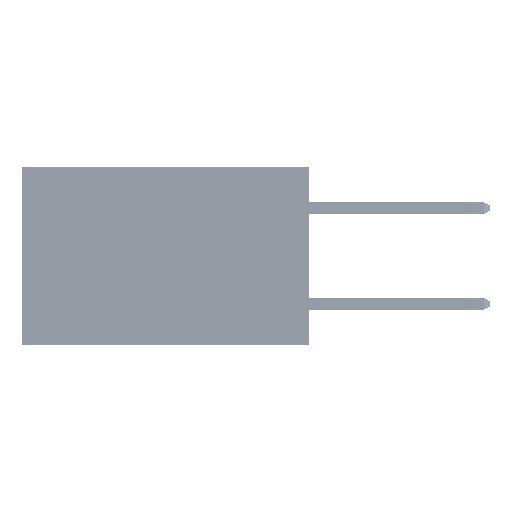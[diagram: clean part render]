
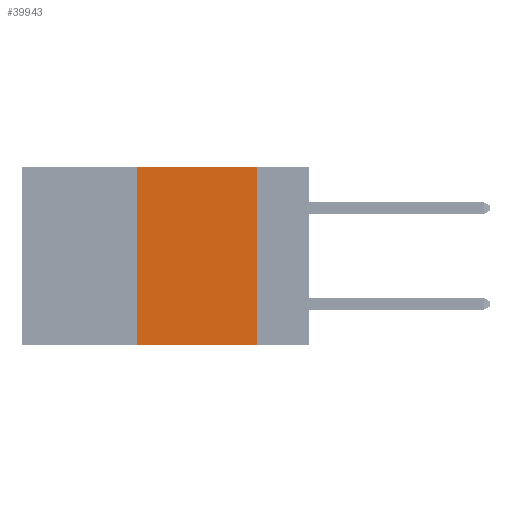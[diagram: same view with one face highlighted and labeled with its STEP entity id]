
A CAD part, left-side view. The second image highlights one B-rep face of the part: STEP entity #39943.
In plain terms, the highlighted planar face has unit normal (-1, 0, 0).
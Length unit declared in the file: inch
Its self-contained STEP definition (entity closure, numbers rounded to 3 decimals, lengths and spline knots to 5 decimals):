
#346 = ORIENTED_EDGE ( 'NONE', *, *, #14190, .F. ) ;
#1102 = VERTEX_POINT ( 'NONE', #16699 ) ;
#1787 = DIRECTION ( 'NONE',  ( 0., 0., -1. ) ) ;
#3929 = AXIS2_PLACEMENT_3D ( 'NONE', #20091, #16231, #43845 ) ;
#5453 = VERTEX_POINT ( 'NONE', #39132 ) ;
#7000 = LINE ( 'NONE', #47631, #37376 ) ;
#9841 = CARTESIAN_POINT ( 'NONE',  ( 0., 0.11, 0. ) ) ;
#10837 = VERTEX_POINT ( 'NONE', #27097 ) ;
#14190 = EDGE_CURVE ( 'NONE', #10837, #29633, #47298, .T. ) ;
#14704 = ORIENTED_EDGE ( 'NONE', *, *, #35596, .T. ) ;
#15706 = DIRECTION ( 'NONE',  ( 0., -1., 0. ) ) ;
#15838 = VECTOR ( 'NONE', #50780, 39.37008 ) ;
#16231 = DIRECTION ( 'NONE',  ( 1., 0., 0. ) ) ;
#16336 = FACE_OUTER_BOUND ( 'NONE', #43054, .T. ) ;
#16699 = CARTESIAN_POINT ( 'NONE',  ( 0., 0.11, -0.37 ) ) ;
#18753 = EDGE_CURVE ( 'NONE', #5453, #10837, #7000, .T. ) ;
#20091 = CARTESIAN_POINT ( 'NONE',  ( 0., 0.6, 0. ) ) ;
#21729 = LINE ( 'NONE', #35399, #30976 ) ;
#24041 = LINE ( 'NONE', #9841, #33251 ) ;
#24071 = ORIENTED_EDGE ( 'NONE', *, *, #18753, .F. ) ;
#25742 = EDGE_CURVE ( 'NONE', #29633, #1102, #24041, .T. ) ;
#27097 = CARTESIAN_POINT ( 'NONE',  ( 0., 0.36, 0. ) ) ;
#29633 = VERTEX_POINT ( 'NONE', #31015 ) ;
#30976 = VECTOR ( 'NONE', #15706, 39.37008 ) ;
#31015 = CARTESIAN_POINT ( 'NONE',  ( 0., 0.11, 0. ) ) ;
#33251 = VECTOR ( 'NONE', #1787, 39.37008 ) ;
#35399 = CARTESIAN_POINT ( 'NONE',  ( 0., 0.6, -0.37 ) ) ;
#35596 = EDGE_CURVE ( 'NONE', #5453, #1102, #21729, .T. ) ;
#35781 = DIRECTION ( 'NONE',  ( 0., 0., 1. ) ) ;
#37376 = VECTOR ( 'NONE', #35781, 39.37008 ) ;
#39132 = CARTESIAN_POINT ( 'NONE',  ( 0., 0.36, -0.37 ) ) ;
#39924 = PLANE ( 'NONE',  #3929 ) ;
#39943 = ADVANCED_FACE ( 'NONE', ( #16336 ), #39924, .F. ) ;
#41898 = ORIENTED_EDGE ( 'NONE', *, *, #25742, .F. ) ;
#42927 = CARTESIAN_POINT ( 'NONE',  ( 0., 0.6, 0. ) ) ;
#43054 = EDGE_LOOP ( 'NONE', ( #41898, #346, #24071, #14704 ) ) ;
#43845 = DIRECTION ( 'NONE',  ( 0., 0., -1. ) ) ;
#47298 = LINE ( 'NONE', #42927, #15838 ) ;
#47631 = CARTESIAN_POINT ( 'NONE',  ( 0., 0.36, 0. ) ) ;
#50780 = DIRECTION ( 'NONE',  ( 0., -1., 0. ) ) ;
